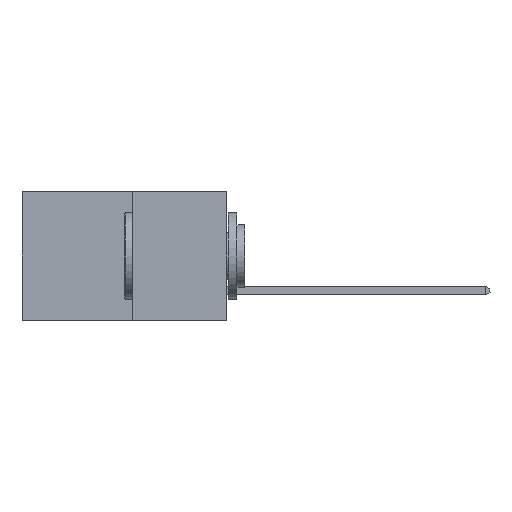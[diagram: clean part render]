
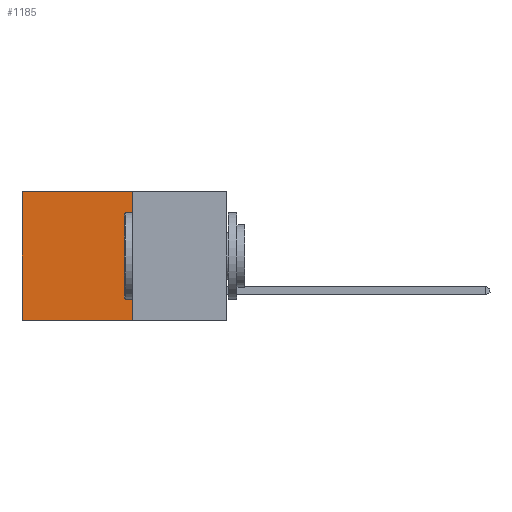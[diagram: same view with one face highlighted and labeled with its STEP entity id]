
A CAD part, left-side view. The second image highlights one B-rep face of the part: STEP entity #1185.
In plain terms, the highlighted planar face has unit normal (-1, 0, 0).
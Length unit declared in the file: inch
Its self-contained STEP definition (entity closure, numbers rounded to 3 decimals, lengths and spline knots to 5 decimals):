
#349 = CARTESIAN_POINT ( 'NONE',  ( 0.277, 0.59, -0.37 ) ) ;
#558 = CARTESIAN_POINT ( 'NONE',  ( 0.277, 0.27, 0. ) ) ;
#660 = DIRECTION ( 'NONE',  ( 1., 0., 0. ) ) ;
#1100 = CARTESIAN_POINT ( 'NONE',  ( 0.277, 0.27, -0.37 ) ) ;
#1131 = VECTOR ( 'NONE', #6035, 39.37008 ) ;
#1185 = ADVANCED_FACE ( 'NONE', ( #8615 ), #6974, .F. ) ;
#1793 = CARTESIAN_POINT ( 'NONE',  ( 0.277, 0.27, -0.37 ) ) ;
#1935 = CARTESIAN_POINT ( 'NONE',  ( 0.277, 0.59, 0. ) ) ;
#2031 = VERTEX_POINT ( 'NONE', #1100 ) ;
#2195 = ORIENTED_EDGE ( 'NONE', *, *, #7387, .F. ) ;
#2583 = DIRECTION ( 'NONE',  ( 0., 1., 0. ) ) ;
#3542 = EDGE_CURVE ( 'NONE', #5842, #5076, #7113, .T. ) ;
#3738 = DIRECTION ( 'NONE',  ( 0., 0., -1. ) ) ;
#4369 = CARTESIAN_POINT ( 'NONE',  ( 0.277, 0.27, -0.37 ) ) ;
#4721 = ORIENTED_EDGE ( 'NONE', *, *, #3542, .T. ) ;
#5004 = VERTEX_POINT ( 'NONE', #349 ) ;
#5041 = LINE ( 'NONE', #4369, #8747 ) ;
#5076 = VERTEX_POINT ( 'NONE', #1935 ) ;
#5111 = AXIS2_PLACEMENT_3D ( 'NONE', #6937, #660, #3738 ) ;
#5842 = VERTEX_POINT ( 'NONE', #558 ) ;
#5871 = ORIENTED_EDGE ( 'NONE', *, *, #7997, .T. ) ;
#6035 = DIRECTION ( 'NONE',  ( 0., 1., 0. ) ) ;
#6132 = LINE ( 'NONE', #1793, #8092 ) ;
#6474 = VECTOR ( 'NONE', #7538, 39.37008 ) ;
#6700 = CARTESIAN_POINT ( 'NONE',  ( 0.277, 0.27, 0. ) ) ;
#6716 = LINE ( 'NONE', #6787, #6474 ) ;
#6787 = CARTESIAN_POINT ( 'NONE',  ( 0.277, 0.59, -0.37 ) ) ;
#6937 = CARTESIAN_POINT ( 'NONE',  ( 0.277, 0.27, -0.37 ) ) ;
#6974 = PLANE ( 'NONE',  #5111 ) ;
#7113 = LINE ( 'NONE', #6700, #1131 ) ;
#7372 = DIRECTION ( 'NONE',  ( 0., 0., -1. ) ) ;
#7387 = EDGE_CURVE ( 'NONE', #2031, #5004, #6132, .T. ) ;
#7538 = DIRECTION ( 'NONE',  ( 0., 0., -1. ) ) ;
#7997 = EDGE_CURVE ( 'NONE', #5076, #5004, #6716, .T. ) ;
#8092 = VECTOR ( 'NONE', #2583, 39.37008 ) ;
#8615 = FACE_OUTER_BOUND ( 'NONE', #9537, .T. ) ;
#8747 = VECTOR ( 'NONE', #7372, 39.37008 ) ;
#9463 = ORIENTED_EDGE ( 'NONE', *, *, #9646, .F. ) ;
#9537 = EDGE_LOOP ( 'NONE', ( #5871, #2195, #9463, #4721 ) ) ;
#9646 = EDGE_CURVE ( 'NONE', #5842, #2031, #5041, .T. ) ;
